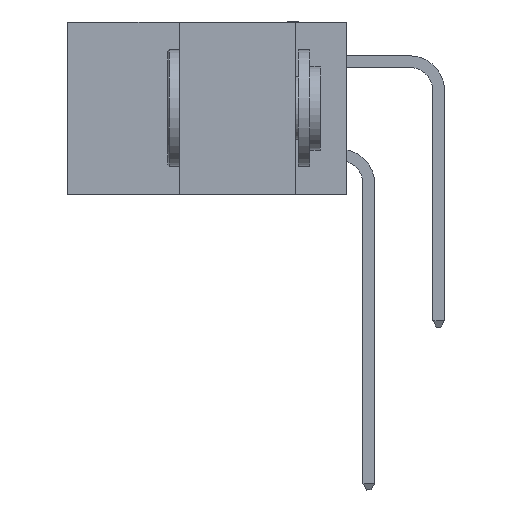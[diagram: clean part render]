
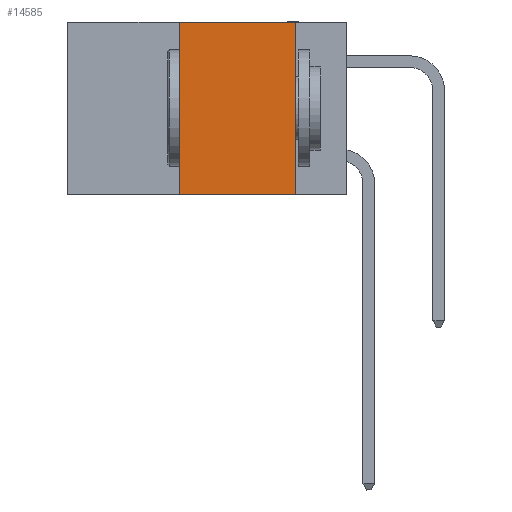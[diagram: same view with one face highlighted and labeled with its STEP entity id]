
A CAD part, left-side view. The second image highlights one B-rep face of the part: STEP entity #14585.
In plain terms, the highlighted planar face has unit normal (-1, 0, 0).
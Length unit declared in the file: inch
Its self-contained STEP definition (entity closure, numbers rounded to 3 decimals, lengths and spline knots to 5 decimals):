
#1757 = VERTEX_POINT ( 'NONE', #32928 ) ;
#2570 = CARTESIAN_POINT ( 'NONE',  ( 0., 0.6, -0.37 ) ) ;
#2594 = LINE ( 'NONE', #17835, #36572 ) ;
#4922 = VERTEX_POINT ( 'NONE', #21029 ) ;
#5154 = VERTEX_POINT ( 'NONE', #15853 ) ;
#5357 = ORIENTED_EDGE ( 'NONE', *, *, #30581, .F. ) ;
#5358 = LINE ( 'NONE', #38536, #13226 ) ;
#6104 = CARTESIAN_POINT ( 'NONE',  ( 0., 0.6, 0. ) ) ;
#8399 = DIRECTION ( 'NONE',  ( 0., -1., 0. ) ) ;
#9787 = DIRECTION ( 'NONE',  ( 0., 0., -1. ) ) ;
#10493 = ORIENTED_EDGE ( 'NONE', *, *, #41407, .F. ) ;
#11097 = ORIENTED_EDGE ( 'NONE', *, *, #35692, .F. ) ;
#13226 = VECTOR ( 'NONE', #22449, 39.37008 ) ;
#14585 = ADVANCED_FACE ( 'NONE', ( #19723 ), #22952, .F. ) ;
#15853 = CARTESIAN_POINT ( 'NONE',  ( 0., 0.36, -0.37 ) ) ;
#17835 = CARTESIAN_POINT ( 'NONE',  ( 0., 0.11, 0. ) ) ;
#18017 = VERTEX_POINT ( 'NONE', #25110 ) ;
#19723 = FACE_OUTER_BOUND ( 'NONE', #26492, .T. ) ;
#21029 = CARTESIAN_POINT ( 'NONE',  ( 0., 0.11, 0. ) ) ;
#22449 = DIRECTION ( 'NONE',  ( 0., 0., 1. ) ) ;
#22575 = DIRECTION ( 'NONE',  ( 0., -1., 0. ) ) ;
#22952 = PLANE ( 'NONE',  #29869 ) ;
#23698 = LINE ( 'NONE', #28082, #41849 ) ;
#24420 = DIRECTION ( 'NONE',  ( 0., 0., -1. ) ) ;
#25110 = CARTESIAN_POINT ( 'NONE',  ( 0., 0.36, 0. ) ) ;
#26492 = EDGE_LOOP ( 'NONE', ( #5357, #11097, #10493, #37544 ) ) ;
#28082 = CARTESIAN_POINT ( 'NONE',  ( 0., 0.6, 0. ) ) ;
#29410 = DIRECTION ( 'NONE',  ( 1., 0., 0. ) ) ;
#29869 = AXIS2_PLACEMENT_3D ( 'NONE', #6104, #29410, #9787 ) ;
#30010 = EDGE_CURVE ( 'NONE', #5154, #1757, #33074, .T. ) ;
#30581 = EDGE_CURVE ( 'NONE', #4922, #1757, #2594, .T. ) ;
#32928 = CARTESIAN_POINT ( 'NONE',  ( 0., 0.11, -0.37 ) ) ;
#33074 = LINE ( 'NONE', #2570, #40668 ) ;
#35692 = EDGE_CURVE ( 'NONE', #18017, #4922, #23698, .T. ) ;
#36572 = VECTOR ( 'NONE', #24420, 39.37008 ) ;
#37544 = ORIENTED_EDGE ( 'NONE', *, *, #30010, .T. ) ;
#38536 = CARTESIAN_POINT ( 'NONE',  ( 0., 0.36, 0. ) ) ;
#40668 = VECTOR ( 'NONE', #22575, 39.37008 ) ;
#41407 = EDGE_CURVE ( 'NONE', #5154, #18017, #5358, .T. ) ;
#41849 = VECTOR ( 'NONE', #8399, 39.37008 ) ;
